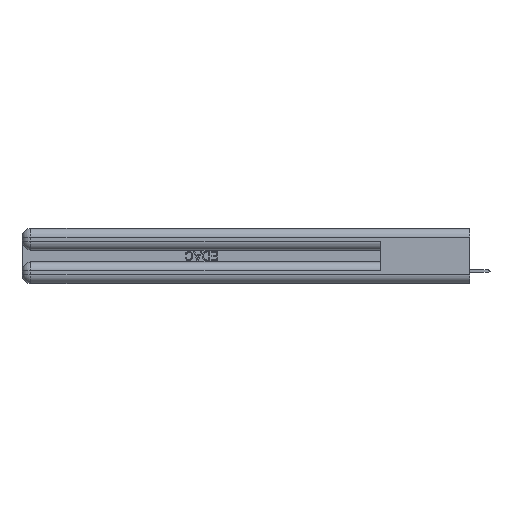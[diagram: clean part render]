
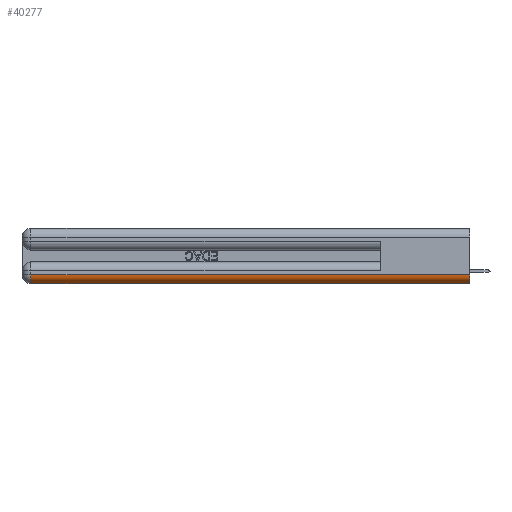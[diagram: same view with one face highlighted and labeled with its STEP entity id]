
A CAD part, left-side view. The second image highlights one B-rep face of the part: STEP entity #40277.
In plain terms, the highlighted cylindrical face has radius 1.524 mm (diameter 3.048 mm), a partial arc.
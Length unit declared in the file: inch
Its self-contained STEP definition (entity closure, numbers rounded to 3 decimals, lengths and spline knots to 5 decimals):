
#214 = LINE ( 'NONE', #32804, #5729 ) ;
#1230 = ORIENTED_EDGE ( 'NONE', *, *, #37336, .F. ) ;
#1471 = ORIENTED_EDGE ( 'NONE', *, *, #28719, .F. ) ;
#4044 = LINE ( 'NONE', #46989, #24980 ) ;
#5729 = VECTOR ( 'NONE', #6897, 39.37008 ) ;
#6897 = DIRECTION ( 'NONE',  ( 0., 1., 0. ) ) ;
#7598 = EDGE_CURVE ( 'NONE', #35365, #27564, #214, .T. ) ;
#7888 = AXIS2_PLACEMENT_3D ( 'NONE', #26625, #8637, #23025 ) ;
#8032 = CARTESIAN_POINT ( 'NONE',  ( 0.06, 2.94, 0. ) ) ;
#8637 = DIRECTION ( 'NONE',  ( 0., 1., 0. ) ) ;
#14150 = FACE_OUTER_BOUND ( 'NONE', #45068, .T. ) ;
#14842 = CARTESIAN_POINT ( 'NONE',  ( 0.06, 0., 0.06 ) ) ;
#15992 = EDGE_CURVE ( 'NONE', #27564, #35001, #17053, .T. ) ;
#17053 = CIRCLE ( 'NONE', #7888, 0.06 ) ;
#17265 = ORIENTED_EDGE ( 'NONE', *, *, #15992, .F. ) ;
#17549 = DIRECTION ( 'NONE',  ( 0., 0., 1. ) ) ;
#17911 = AXIS2_PLACEMENT_3D ( 'NONE', #14842, #25178, #18220 ) ;
#18220 = DIRECTION ( 'NONE',  ( 0., 0., 1. ) ) ;
#20068 = CARTESIAN_POINT ( 'NONE',  ( 0.06, 0., 0. ) ) ;
#20252 = ORIENTED_EDGE ( 'NONE', *, *, #7598, .F. ) ;
#21568 = AXIS2_PLACEMENT_3D ( 'NONE', #28808, #24508, #17549 ) ;
#23025 = DIRECTION ( 'NONE',  ( 0., 0., 1. ) ) ;
#24508 = DIRECTION ( 'NONE',  ( 0., -1., 0. ) ) ;
#24980 = VECTOR ( 'NONE', #33284, 39.37008 ) ;
#25178 = DIRECTION ( 'NONE',  ( 0., 1., 0. ) ) ;
#26625 = CARTESIAN_POINT ( 'NONE',  ( 0.06, 2.94, 0.06 ) ) ;
#27564 = VERTEX_POINT ( 'NONE', #8032 ) ;
#28490 = CIRCLE ( 'NONE', #21568, 0.06 ) ;
#28719 = EDGE_CURVE ( 'NONE', #35001, #29782, #4044, .T. ) ;
#28808 = CARTESIAN_POINT ( 'NONE',  ( 0.06, 0., 0.06 ) ) ;
#29782 = VERTEX_POINT ( 'NONE', #45828 ) ;
#32804 = CARTESIAN_POINT ( 'NONE',  ( 0.06, 3., 0. ) ) ;
#33284 = DIRECTION ( 'NONE',  ( 0., -1., 0. ) ) ;
#35001 = VERTEX_POINT ( 'NONE', #42894 ) ;
#35365 = VERTEX_POINT ( 'NONE', #20068 ) ;
#37336 = EDGE_CURVE ( 'NONE', #29782, #35365, #28490, .T. ) ;
#40277 = ADVANCED_FACE ( 'NONE', ( #14150 ), #43880, .T. ) ;
#42894 = CARTESIAN_POINT ( 'NONE',  ( 0., 2.94, 0.06 ) ) ;
#43880 = CYLINDRICAL_SURFACE ( 'NONE', #17911, 0.06 ) ;
#45068 = EDGE_LOOP ( 'NONE', ( #1230, #1471, #17265, #20252 ) ) ;
#45828 = CARTESIAN_POINT ( 'NONE',  ( 0., 0., 0.06 ) ) ;
#46989 = CARTESIAN_POINT ( 'NONE',  ( 0., 0., 0.06 ) ) ;
